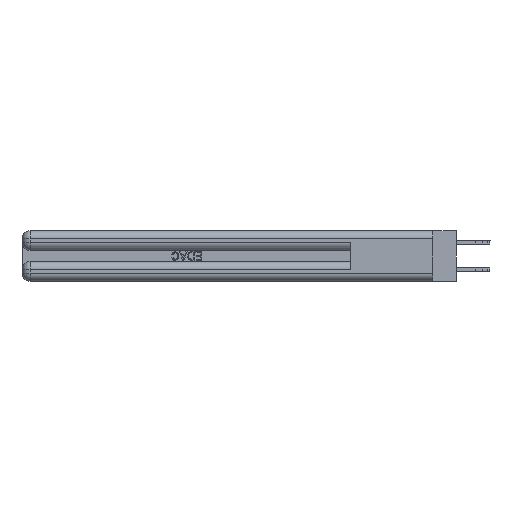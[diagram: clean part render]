
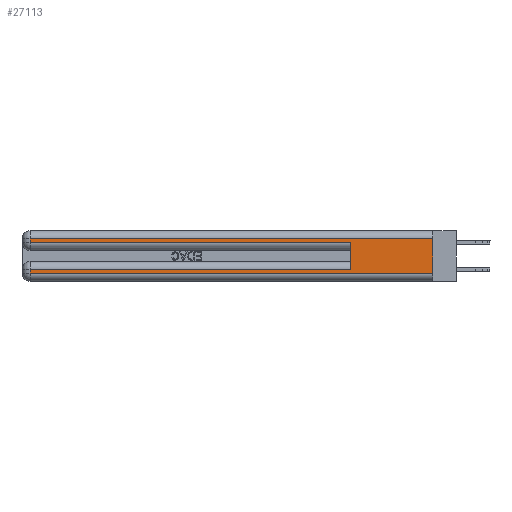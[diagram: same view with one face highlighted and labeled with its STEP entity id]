
A CAD part, left-side view. The second image highlights one B-rep face of the part: STEP entity #27113.
In plain terms, the highlighted planar face has unit normal (-1, 0, 0).
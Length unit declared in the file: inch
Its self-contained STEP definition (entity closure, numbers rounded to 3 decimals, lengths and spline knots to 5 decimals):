
#754 = ORIENTED_EDGE ( 'NONE', *, *, #25974, .T. ) ;
#969 = EDGE_CURVE ( 'NONE', #16858, #20067, #24722, .T. ) ;
#1042 = ORIENTED_EDGE ( 'NONE', *, *, #30187, .F. ) ;
#1328 = VERTEX_POINT ( 'NONE', #34140 ) ;
#1355 = LINE ( 'NONE', #12433, #30370 ) ;
#2420 = EDGE_CURVE ( 'NONE', #1328, #35477, #8518, .T. ) ;
#2498 = CARTESIAN_POINT ( 'NONE',  ( 0., 0., 0.06 ) ) ;
#3012 = LINE ( 'NONE', #14197, #35996 ) ;
#3108 = VECTOR ( 'NONE', #10474, 39.37008 ) ;
#4431 = PLANE ( 'NONE',  #8424 ) ;
#5079 = CARTESIAN_POINT ( 'NONE',  ( 0., 2.94, 0.31 ) ) ;
#5789 = VERTEX_POINT ( 'NONE', #9439 ) ;
#6772 = ORIENTED_EDGE ( 'NONE', *, *, #20940, .F. ) ;
#7845 = DIRECTION ( 'NONE',  ( 0., 0., -1. ) ) ;
#8223 = CARTESIAN_POINT ( 'NONE',  ( 0., 0.6, 0.285 ) ) ;
#8424 = AXIS2_PLACEMENT_3D ( 'NONE', #26492, #36481, #39113 ) ;
#8518 = LINE ( 'NONE', #8890, #38587 ) ;
#8625 = DIRECTION ( 'NONE',  ( 0., -1., 0. ) ) ;
#8817 = CARTESIAN_POINT ( 'NONE',  ( 0., 2.94, 0.285 ) ) ;
#8890 = CARTESIAN_POINT ( 'NONE',  ( 0., 0., 0.31 ) ) ;
#9439 = CARTESIAN_POINT ( 'NONE',  ( 0., 2.94, 0.085 ) ) ;
#9544 = CARTESIAN_POINT ( 'NONE',  ( 0., 0., 0.085 ) ) ;
#9681 = DIRECTION ( 'NONE',  ( 0., 1., 0. ) ) ;
#10474 = DIRECTION ( 'NONE',  ( 0., 0., -1. ) ) ;
#10807 = CARTESIAN_POINT ( 'NONE',  ( 0., 2.94, 0.37 ) ) ;
#11072 = ORIENTED_EDGE ( 'NONE', *, *, #2420, .T. ) ;
#11473 = EDGE_CURVE ( 'NONE', #35477, #15682, #12587, .T. ) ;
#11566 = VECTOR ( 'NONE', #9681, 39.37008 ) ;
#12433 = CARTESIAN_POINT ( 'NONE',  ( 0., 0., 0.285 ) ) ;
#12510 = VERTEX_POINT ( 'NONE', #8223 ) ;
#12587 = LINE ( 'NONE', #10807, #3108 ) ;
#12800 = DIRECTION ( 'NONE',  ( 0., 0., 1. ) ) ;
#13125 = VECTOR ( 'NONE', #12800, 39.37008 ) ;
#14197 = CARTESIAN_POINT ( 'NONE',  ( 0., 0., 0.37 ) ) ;
#15616 = DIRECTION ( 'NONE',  ( 0., 1., 0. ) ) ;
#15682 = VERTEX_POINT ( 'NONE', #8817 ) ;
#16858 = VERTEX_POINT ( 'NONE', #40754 ) ;
#17377 = CARTESIAN_POINT ( 'NONE',  ( 0., 2.94, 0.37 ) ) ;
#19665 = LINE ( 'NONE', #38282, #13125 ) ;
#20067 = VERTEX_POINT ( 'NONE', #2498 ) ;
#20940 = EDGE_CURVE ( 'NONE', #1328, #20067, #3012, .T. ) ;
#23099 = LINE ( 'NONE', #9544, #11566 ) ;
#24722 = LINE ( 'NONE', #38205, #27183 ) ;
#24746 = DIRECTION ( 'NONE',  ( 0., -1., 0. ) ) ;
#25238 = VECTOR ( 'NONE', #7845, 39.37008 ) ;
#25792 = CARTESIAN_POINT ( 'NONE',  ( 0., 0.6, 0.085 ) ) ;
#25974 = EDGE_CURVE ( 'NONE', #5789, #16858, #33718, .T. ) ;
#26492 = CARTESIAN_POINT ( 'NONE',  ( 0., 0., 0.37 ) ) ;
#26921 = DIRECTION ( 'NONE',  ( 0., 0., -1. ) ) ;
#27113 = ADVANCED_FACE ( 'NONE', ( #37141 ), #4431, .F. ) ;
#27183 = VECTOR ( 'NONE', #24746, 39.37008 ) ;
#28135 = EDGE_CURVE ( 'NONE', #37886, #5789, #23099, .T. ) ;
#30187 = EDGE_CURVE ( 'NONE', #37886, #12510, #19665, .T. ) ;
#30370 = VECTOR ( 'NONE', #8625, 39.37008 ) ;
#30868 = EDGE_LOOP ( 'NONE', ( #6772, #11072, #33846, #35340, #1042, #40983, #754, #35512 ) ) ;
#33718 = LINE ( 'NONE', #17377, #25238 ) ;
#33846 = ORIENTED_EDGE ( 'NONE', *, *, #11473, .T. ) ;
#34140 = CARTESIAN_POINT ( 'NONE',  ( 0., 0., 0.31 ) ) ;
#35340 = ORIENTED_EDGE ( 'NONE', *, *, #41472, .T. ) ;
#35477 = VERTEX_POINT ( 'NONE', #5079 ) ;
#35512 = ORIENTED_EDGE ( 'NONE', *, *, #969, .T. ) ;
#35996 = VECTOR ( 'NONE', #26921, 39.37008 ) ;
#36481 = DIRECTION ( 'NONE',  ( 1., 0., 0. ) ) ;
#37141 = FACE_OUTER_BOUND ( 'NONE', #30868, .T. ) ;
#37886 = VERTEX_POINT ( 'NONE', #25792 ) ;
#38205 = CARTESIAN_POINT ( 'NONE',  ( 0., 0., 0.06 ) ) ;
#38282 = CARTESIAN_POINT ( 'NONE',  ( 0., 0.6, 0.145 ) ) ;
#38587 = VECTOR ( 'NONE', #15616, 39.37008 ) ;
#39113 = DIRECTION ( 'NONE',  ( 0., 0., -1. ) ) ;
#40754 = CARTESIAN_POINT ( 'NONE',  ( 0., 2.94, 0.06 ) ) ;
#40983 = ORIENTED_EDGE ( 'NONE', *, *, #28135, .T. ) ;
#41472 = EDGE_CURVE ( 'NONE', #15682, #12510, #1355, .T. ) ;
